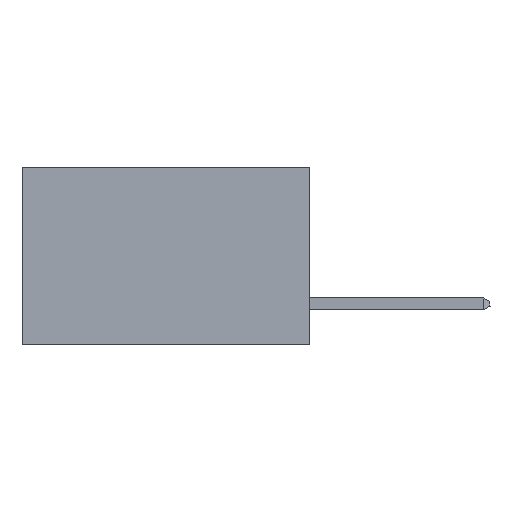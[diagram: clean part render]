
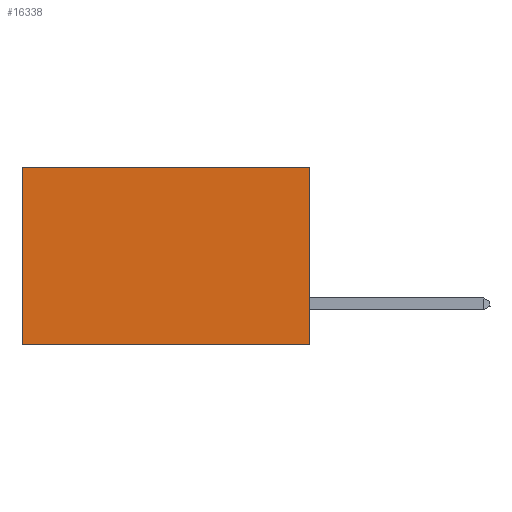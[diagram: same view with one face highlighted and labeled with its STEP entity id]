
A CAD part, left-side view. The second image highlights one B-rep face of the part: STEP entity #16338.
In plain terms, the highlighted planar face has unit normal (-1, 0, 0).
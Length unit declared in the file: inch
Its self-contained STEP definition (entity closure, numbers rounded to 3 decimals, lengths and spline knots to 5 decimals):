
#514 = LINE ( 'NONE', #4051, #11250 ) ;
#797 = VECTOR ( 'NONE', #9464, 39.37008 ) ;
#1468 = LINE ( 'NONE', #11635, #797 ) ;
#1536 = DIRECTION ( 'NONE',  ( 0., 1., 0. ) ) ;
#1738 = DIRECTION ( 'NONE',  ( 0., 0., -1. ) ) ;
#2950 = EDGE_CURVE ( 'NONE', #15817, #7562, #514, .T. ) ;
#4051 = CARTESIAN_POINT ( 'NONE',  ( 0.2875, 0., -0.37 ) ) ;
#5051 = VECTOR ( 'NONE', #9550, 39.37008 ) ;
#7407 = EDGE_CURVE ( 'NONE', #9477, #7562, #17715, .T. ) ;
#7562 = VERTEX_POINT ( 'NONE', #14405 ) ;
#8329 = CARTESIAN_POINT ( 'NONE',  ( 0.2875, 0., 0. ) ) ;
#9464 = DIRECTION ( 'NONE',  ( 0., 1., 0. ) ) ;
#9477 = VERTEX_POINT ( 'NONE', #26662 ) ;
#9550 = DIRECTION ( 'NONE',  ( 0., 0., -1. ) ) ;
#9835 = AXIS2_PLACEMENT_3D ( 'NONE', #26743, #14582, #1738 ) ;
#10361 = VERTEX_POINT ( 'NONE', #8329 ) ;
#11240 = ORIENTED_EDGE ( 'NONE', *, *, #27001, .F. ) ;
#11250 = VECTOR ( 'NONE', #1536, 39.37008 ) ;
#11469 = EDGE_LOOP ( 'NONE', ( #12239, #12620, #11240, #15699 ) ) ;
#11635 = CARTESIAN_POINT ( 'NONE',  ( 0.2875, 0., 0. ) ) ;
#11719 = CARTESIAN_POINT ( 'NONE',  ( 0.2875, 0.6, 0. ) ) ;
#12019 = EDGE_CURVE ( 'NONE', #10361, #9477, #1468, .T. ) ;
#12239 = ORIENTED_EDGE ( 'NONE', *, *, #7407, .T. ) ;
#12620 = ORIENTED_EDGE ( 'NONE', *, *, #2950, .F. ) ;
#12871 = DIRECTION ( 'NONE',  ( 0., 0., -1. ) ) ;
#14303 = VECTOR ( 'NONE', #12871, 39.37008 ) ;
#14405 = CARTESIAN_POINT ( 'NONE',  ( 0.2875, 0.6, -0.37 ) ) ;
#14582 = DIRECTION ( 'NONE',  ( 1., 0., 0. ) ) ;
#15699 = ORIENTED_EDGE ( 'NONE', *, *, #12019, .T. ) ;
#15817 = VERTEX_POINT ( 'NONE', #20820 ) ;
#16338 = ADVANCED_FACE ( 'NONE', ( #25014 ), #16581, .F. ) ;
#16581 = PLANE ( 'NONE',  #9835 ) ;
#17715 = LINE ( 'NONE', #11719, #5051 ) ;
#20820 = CARTESIAN_POINT ( 'NONE',  ( 0.2875, 0., -0.37 ) ) ;
#23245 = LINE ( 'NONE', #25134, #14303 ) ;
#25014 = FACE_OUTER_BOUND ( 'NONE', #11469, .T. ) ;
#25134 = CARTESIAN_POINT ( 'NONE',  ( 0.2875, 0., 0. ) ) ;
#26662 = CARTESIAN_POINT ( 'NONE',  ( 0.2875, 0.6, 0. ) ) ;
#26743 = CARTESIAN_POINT ( 'NONE',  ( 0.2875, 0., 0. ) ) ;
#27001 = EDGE_CURVE ( 'NONE', #10361, #15817, #23245, .T. ) ;
